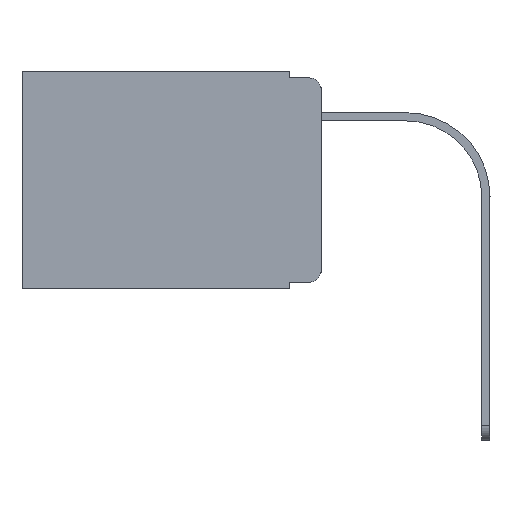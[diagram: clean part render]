
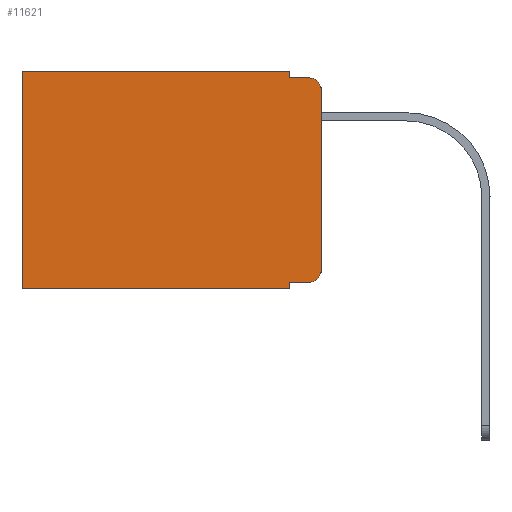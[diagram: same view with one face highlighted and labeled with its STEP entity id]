
A CAD part, left-side view. The second image highlights one B-rep face of the part: STEP entity #11621.
In plain terms, the highlighted planar face has unit normal (-1, 0, 0).
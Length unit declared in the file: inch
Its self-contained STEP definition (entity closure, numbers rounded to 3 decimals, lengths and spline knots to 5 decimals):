
#55 = CARTESIAN_POINT ( 'NONE',  ( 0.298, 0.051, 0. ) ) ;
#168 = VECTOR ( 'NONE', #6530, 39.37008 ) ;
#606 = EDGE_CURVE ( 'NONE', #3806, #8662, #7693, .T. ) ;
#640 = VECTOR ( 'NONE', #5226, 39.37008 ) ;
#925 = EDGE_CURVE ( 'NONE', #5548, #7925, #11671, .T. ) ;
#957 = DIRECTION ( 'NONE',  ( 0., -1., 0. ) ) ;
#1069 = CARTESIAN_POINT ( 'NONE',  ( 0.298, 0.473, 0. ) ) ;
#1483 = EDGE_CURVE ( 'NONE', #4815, #3283, #12248, .T. ) ;
#1777 = CARTESIAN_POINT ( 'NONE',  ( 0.298, 0., 0. ) ) ;
#1881 = CARTESIAN_POINT ( 'NONE',  ( 0.298, 0.051, -0.01 ) ) ;
#2200 = EDGE_CURVE ( 'NONE', #8810, #3283, #6621, .T. ) ;
#2455 = ORIENTED_EDGE ( 'NONE', *, *, #6269, .T. ) ;
#2720 = CARTESIAN_POINT ( 'NONE',  ( 0.298, 0., -0.343 ) ) ;
#2751 = VECTOR ( 'NONE', #5126, 39.37008 ) ;
#2753 = DIRECTION ( 'NONE',  ( 0., 0., -1. ) ) ;
#3114 = VECTOR ( 'NONE', #10643, 39.37008 ) ;
#3283 = VERTEX_POINT ( 'NONE', #11024 ) ;
#3390 = CARTESIAN_POINT ( 'NONE',  ( 0.298, 0.02, -0.03 ) ) ;
#3560 = VERTEX_POINT ( 'NONE', #9894 ) ;
#3806 = VERTEX_POINT ( 'NONE', #11245 ) ;
#4236 = VECTOR ( 'NONE', #4574, 39.37008 ) ;
#4446 = AXIS2_PLACEMENT_3D ( 'NONE', #3390, #7081, #7204 ) ;
#4482 = CARTESIAN_POINT ( 'NONE',  ( 0.298, 0.02, -0.333 ) ) ;
#4574 = DIRECTION ( 'NONE',  ( 0., 0., -1. ) ) ;
#4578 = CARTESIAN_POINT ( 'NONE',  ( 0.298, 0.051, -0.343 ) ) ;
#4595 = ORIENTED_EDGE ( 'NONE', *, *, #10855, .T. ) ;
#4815 = VERTEX_POINT ( 'NONE', #5931 ) ;
#5126 = DIRECTION ( 'NONE',  ( 0., 0., -1. ) ) ;
#5198 = ORIENTED_EDGE ( 'NONE', *, *, #1483, .T. ) ;
#5226 = DIRECTION ( 'NONE',  ( 0., 0., -1. ) ) ;
#5494 = DIRECTION ( 'NONE',  ( 0., -1., 0. ) ) ;
#5548 = VERTEX_POINT ( 'NONE', #55 ) ;
#5585 = DIRECTION ( 'NONE',  ( 1., 0., 0. ) ) ;
#5594 = EDGE_CURVE ( 'NONE', #8662, #10322, #11294, .T. ) ;
#5862 = LINE ( 'NONE', #8054, #4236 ) ;
#5931 = CARTESIAN_POINT ( 'NONE',  ( 0.298, 0., -0.03 ) ) ;
#6099 = ORIENTED_EDGE ( 'NONE', *, *, #11377, .F. ) ;
#6269 = EDGE_CURVE ( 'NONE', #7925, #10322, #9778, .T. ) ;
#6471 = VECTOR ( 'NONE', #5494, 39.37008 ) ;
#6518 = FACE_OUTER_BOUND ( 'NONE', #10310, .T. ) ;
#6530 = DIRECTION ( 'NONE',  ( 0., 1., 0. ) ) ;
#6621 = LINE ( 'NONE', #1881, #6471 ) ;
#6759 = VECTOR ( 'NONE', #8726, 39.37008 ) ;
#7081 = DIRECTION ( 'NONE',  ( -1., 0., 0. ) ) ;
#7204 = DIRECTION ( 'NONE',  ( 0., 0., -1. ) ) ;
#7503 = DIRECTION ( 'NONE',  ( -1., 0., 0. ) ) ;
#7620 = ORIENTED_EDGE ( 'NONE', *, *, #5594, .F. ) ;
#7693 = LINE ( 'NONE', #9650, #3114 ) ;
#7925 = VERTEX_POINT ( 'NONE', #1069 ) ;
#7942 = CARTESIAN_POINT ( 'NONE',  ( 0.298, 0.473, 0. ) ) ;
#8027 = CIRCLE ( 'NONE', #10231, 0.02 ) ;
#8054 = CARTESIAN_POINT ( 'NONE',  ( 0.298, 0., 0. ) ) ;
#8437 = AXIS2_PLACEMENT_3D ( 'NONE', #1777, #5585, #12281 ) ;
#8662 = VERTEX_POINT ( 'NONE', #4578 ) ;
#8726 = DIRECTION ( 'NONE',  ( 0., 1., 0. ) ) ;
#8810 = VERTEX_POINT ( 'NONE', #9673 ) ;
#9394 = CARTESIAN_POINT ( 'NONE',  ( 0.298, 0.02, -0.313 ) ) ;
#9423 = ORIENTED_EDGE ( 'NONE', *, *, #9859, .F. ) ;
#9435 = ORIENTED_EDGE ( 'NONE', *, *, #2200, .F. ) ;
#9522 = CARTESIAN_POINT ( 'NONE',  ( 0.298, 0.051, -0.333 ) ) ;
#9650 = CARTESIAN_POINT ( 'NONE',  ( 0.298, 0.051, 0. ) ) ;
#9673 = CARTESIAN_POINT ( 'NONE',  ( 0.298, 0.051, -0.01 ) ) ;
#9778 = LINE ( 'NONE', #7942, #2751 ) ;
#9859 = EDGE_CURVE ( 'NONE', #5548, #8810, #9992, .T. ) ;
#9894 = CARTESIAN_POINT ( 'NONE',  ( 0.298, 0., -0.313 ) ) ;
#9992 = LINE ( 'NONE', #10991, #640 ) ;
#10025 = VECTOR ( 'NONE', #957, 39.37008 ) ;
#10042 = ORIENTED_EDGE ( 'NONE', *, *, #925, .T. ) ;
#10208 = ORIENTED_EDGE ( 'NONE', *, *, #606, .F. ) ;
#10231 = AXIS2_PLACEMENT_3D ( 'NONE', #9394, #7503, #2753 ) ;
#10310 = EDGE_LOOP ( 'NONE', ( #6099, #5198, #9435, #9423, #10042, #2455, #7620, #10208, #10801, #4595 ) ) ;
#10322 = VERTEX_POINT ( 'NONE', #10473 ) ;
#10348 = PLANE ( 'NONE',  #8437 ) ;
#10473 = CARTESIAN_POINT ( 'NONE',  ( 0.298, 0.473, -0.343 ) ) ;
#10551 = CARTESIAN_POINT ( 'NONE',  ( 0.298, 0., 0. ) ) ;
#10643 = DIRECTION ( 'NONE',  ( 0., 0., -1. ) ) ;
#10801 = ORIENTED_EDGE ( 'NONE', *, *, #10882, .T. ) ;
#10855 = EDGE_CURVE ( 'NONE', #12306, #3560, #8027, .T. ) ;
#10882 = EDGE_CURVE ( 'NONE', #3806, #12306, #11388, .T. ) ;
#10991 = CARTESIAN_POINT ( 'NONE',  ( 0.298, 0.051, 0. ) ) ;
#11024 = CARTESIAN_POINT ( 'NONE',  ( 0.298, 0.02, -0.01 ) ) ;
#11245 = CARTESIAN_POINT ( 'NONE',  ( 0.298, 0.051, -0.333 ) ) ;
#11294 = LINE ( 'NONE', #2720, #168 ) ;
#11377 = EDGE_CURVE ( 'NONE', #4815, #3560, #5862, .T. ) ;
#11388 = LINE ( 'NONE', #9522, #10025 ) ;
#11621 = ADVANCED_FACE ( 'NONE', ( #6518 ), #10348, .F. ) ;
#11671 = LINE ( 'NONE', #10551, #6759 ) ;
#12248 = CIRCLE ( 'NONE', #4446, 0.02 ) ;
#12281 = DIRECTION ( 'NONE',  ( 0., 0., -1. ) ) ;
#12306 = VERTEX_POINT ( 'NONE', #4482 ) ;
